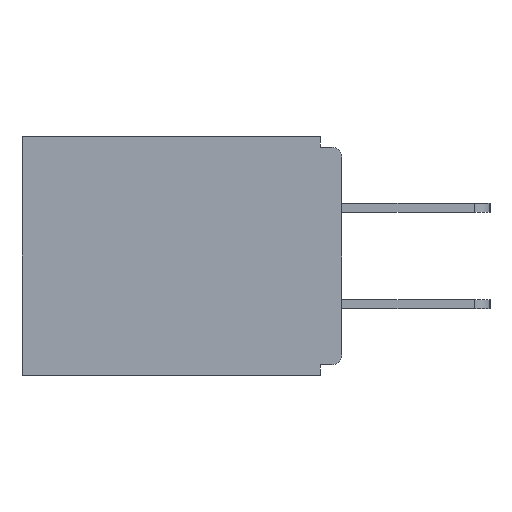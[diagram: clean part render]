
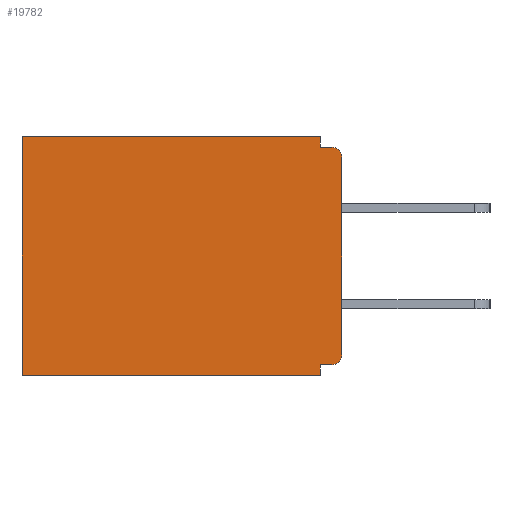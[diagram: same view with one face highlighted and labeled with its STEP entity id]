
A CAD part, left-side view. The second image highlights one B-rep face of the part: STEP entity #19782.
In plain terms, the highlighted planar face has unit normal (-1, 0, 0).
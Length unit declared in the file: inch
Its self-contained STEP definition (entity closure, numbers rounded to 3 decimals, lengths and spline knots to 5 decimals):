
#563 = VERTEX_POINT ( 'NONE', #11566 ) ;
#875 = EDGE_CURVE ( 'NONE', #18219, #6310, #6200, .T. ) ;
#1026 = EDGE_CURVE ( 'NONE', #14572, #13805, #2818, .T. ) ;
#1459 = DIRECTION ( 'NONE',  ( 0., 1., 0. ) ) ;
#1537 = ORIENTED_EDGE ( 'NONE', *, *, #14484, .F. ) ;
#1582 = EDGE_CURVE ( 'NONE', #19949, #13805, #2573, .T. ) ;
#2117 = PLANE ( 'NONE',  #2501 ) ;
#2447 = CARTESIAN_POINT ( 'NONE',  ( 0.298, 0., 0. ) ) ;
#2501 = AXIS2_PLACEMENT_3D ( 'NONE', #6794, #17654, #19233 ) ;
#2573 = LINE ( 'NONE', #12320, #18588 ) ;
#2705 = ORIENTED_EDGE ( 'NONE', *, *, #12603, .F. ) ;
#2717 = CARTESIAN_POINT ( 'NONE',  ( 0.298, 0.015, -0.03 ) ) ;
#2818 = LINE ( 'NONE', #11333, #10050 ) ;
#2831 = LINE ( 'NONE', #13213, #3318 ) ;
#3318 = VECTOR ( 'NONE', #13082, 39.37008 ) ;
#3499 = ORIENTED_EDGE ( 'NONE', *, *, #1026, .T. ) ;
#3520 = DIRECTION ( 'NONE',  ( 0., 0., -1. ) ) ;
#3714 = EDGE_LOOP ( 'NONE', ( #18921, #5028, #9252, #6297, #3499, #17788, #2705, #19686, #15140, #1537 ) ) ;
#3827 = LINE ( 'NONE', #18552, #12309 ) ;
#4015 = DIRECTION ( 'NONE',  ( 0., 0., -1. ) ) ;
#5028 = ORIENTED_EDGE ( 'NONE', *, *, #15859, .F. ) ;
#5349 = CARTESIAN_POINT ( 'NONE',  ( 0.298, 0.46, -0.343 ) ) ;
#5506 = CARTESIAN_POINT ( 'NONE',  ( 0.298, 0.015, -0.015 ) ) ;
#6104 = EDGE_CURVE ( 'NONE', #18219, #563, #6687, .T. ) ;
#6200 = LINE ( 'NONE', #7475, #6696 ) ;
#6297 = ORIENTED_EDGE ( 'NONE', *, *, #15418, .T. ) ;
#6310 = VERTEX_POINT ( 'NONE', #9239 ) ;
#6676 = DIRECTION ( 'NONE',  ( 0., 0., -1. ) ) ;
#6687 = CIRCLE ( 'NONE', #18587, 0.015 ) ;
#6696 = VECTOR ( 'NONE', #1459, 39.37008 ) ;
#6794 = CARTESIAN_POINT ( 'NONE',  ( 0.298, 0., 0. ) ) ;
#7475 = CARTESIAN_POINT ( 'NONE',  ( 0.298, 0., -0.328 ) ) ;
#7769 = LINE ( 'NONE', #18858, #8018 ) ;
#8018 = VECTOR ( 'NONE', #3520, 39.37008 ) ;
#8633 = DIRECTION ( 'NONE',  ( 0., 0., -1. ) ) ;
#9239 = CARTESIAN_POINT ( 'NONE',  ( 0.298, 0.031, -0.328 ) ) ;
#9252 = ORIENTED_EDGE ( 'NONE', *, *, #14466, .F. ) ;
#9434 = VERTEX_POINT ( 'NONE', #12703 ) ;
#9672 = CARTESIAN_POINT ( 'NONE',  ( 0.298, 0.015, -0.313 ) ) ;
#10050 = VECTOR ( 'NONE', #19300, 39.37008 ) ;
#10832 = LINE ( 'NONE', #11974, #12796 ) ;
#10865 = AXIS2_PLACEMENT_3D ( 'NONE', #2717, #11786, #18184 ) ;
#11324 = CIRCLE ( 'NONE', #10865, 0.015 ) ;
#11333 = CARTESIAN_POINT ( 'NONE',  ( 0.298, 0.46, 0. ) ) ;
#11566 = CARTESIAN_POINT ( 'NONE',  ( 0.298, 0., -0.313 ) ) ;
#11786 = DIRECTION ( 'NONE',  ( -1., 0., 0. ) ) ;
#11962 = CARTESIAN_POINT ( 'NONE',  ( 0.298, 0.031, 0. ) ) ;
#11974 = CARTESIAN_POINT ( 'NONE',  ( 0.298, 0.031, -0.343 ) ) ;
#12303 = VECTOR ( 'NONE', #4015, 39.37008 ) ;
#12309 = VECTOR ( 'NONE', #15351, 39.37008 ) ;
#12320 = CARTESIAN_POINT ( 'NONE',  ( 0.298, 0., -0.343 ) ) ;
#12603 = EDGE_CURVE ( 'NONE', #6310, #19949, #7769, .T. ) ;
#12703 = CARTESIAN_POINT ( 'NONE',  ( 0.298, 0., -0.03 ) ) ;
#12796 = VECTOR ( 'NONE', #8633, 39.37008 ) ;
#13082 = DIRECTION ( 'NONE',  ( 0., -1., 0. ) ) ;
#13213 = CARTESIAN_POINT ( 'NONE',  ( 0.298, 0., -0.015 ) ) ;
#13370 = CARTESIAN_POINT ( 'NONE',  ( 0.298, 0.031, -0.343 ) ) ;
#13805 = VERTEX_POINT ( 'NONE', #5349 ) ;
#13947 = VERTEX_POINT ( 'NONE', #11962 ) ;
#14466 = EDGE_CURVE ( 'NONE', #13947, #15211, #10832, .T. ) ;
#14484 = EDGE_CURVE ( 'NONE', #9434, #563, #16454, .T. ) ;
#14513 = EDGE_CURVE ( 'NONE', #9434, #16918, #11324, .T. ) ;
#14572 = VERTEX_POINT ( 'NONE', #18441 ) ;
#15071 = FACE_OUTER_BOUND ( 'NONE', #3714, .T. ) ;
#15140 = ORIENTED_EDGE ( 'NONE', *, *, #6104, .T. ) ;
#15211 = VERTEX_POINT ( 'NONE', #16577 ) ;
#15351 = DIRECTION ( 'NONE',  ( 0., 1., 0. ) ) ;
#15418 = EDGE_CURVE ( 'NONE', #13947, #14572, #3827, .T. ) ;
#15516 = DIRECTION ( 'NONE',  ( 0., 1., 0. ) ) ;
#15859 = EDGE_CURVE ( 'NONE', #15211, #16918, #2831, .T. ) ;
#16454 = LINE ( 'NONE', #2447, #12303 ) ;
#16577 = CARTESIAN_POINT ( 'NONE',  ( 0.298, 0.031, -0.015 ) ) ;
#16918 = VERTEX_POINT ( 'NONE', #5506 ) ;
#17581 = CARTESIAN_POINT ( 'NONE',  ( 0.298, 0.015, -0.328 ) ) ;
#17654 = DIRECTION ( 'NONE',  ( 1., 0., 0. ) ) ;
#17788 = ORIENTED_EDGE ( 'NONE', *, *, #1582, .F. ) ;
#18184 = DIRECTION ( 'NONE',  ( 0., 0., -1. ) ) ;
#18219 = VERTEX_POINT ( 'NONE', #17581 ) ;
#18441 = CARTESIAN_POINT ( 'NONE',  ( 0.298, 0.46, 0. ) ) ;
#18552 = CARTESIAN_POINT ( 'NONE',  ( 0.298, 0., 0. ) ) ;
#18587 = AXIS2_PLACEMENT_3D ( 'NONE', #9672, #19035, #6676 ) ;
#18588 = VECTOR ( 'NONE', #15516, 39.37008 ) ;
#18858 = CARTESIAN_POINT ( 'NONE',  ( 0.298, 0.031, -0.343 ) ) ;
#18921 = ORIENTED_EDGE ( 'NONE', *, *, #14513, .T. ) ;
#19035 = DIRECTION ( 'NONE',  ( -1., 0., 0. ) ) ;
#19233 = DIRECTION ( 'NONE',  ( 0., 0., -1. ) ) ;
#19300 = DIRECTION ( 'NONE',  ( 0., 0., -1. ) ) ;
#19686 = ORIENTED_EDGE ( 'NONE', *, *, #875, .F. ) ;
#19782 = ADVANCED_FACE ( 'NONE', ( #15071 ), #2117, .F. ) ;
#19949 = VERTEX_POINT ( 'NONE', #13370 ) ;
